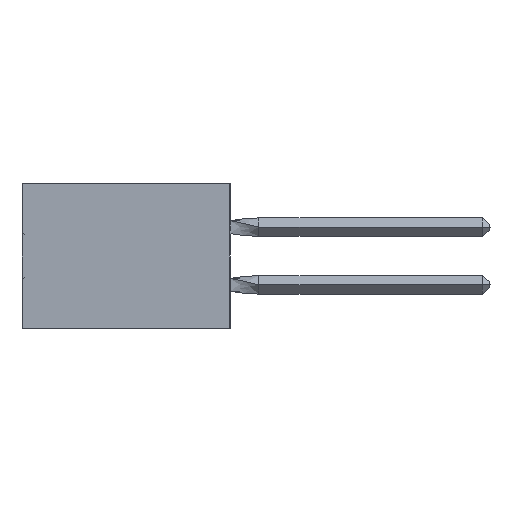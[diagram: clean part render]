
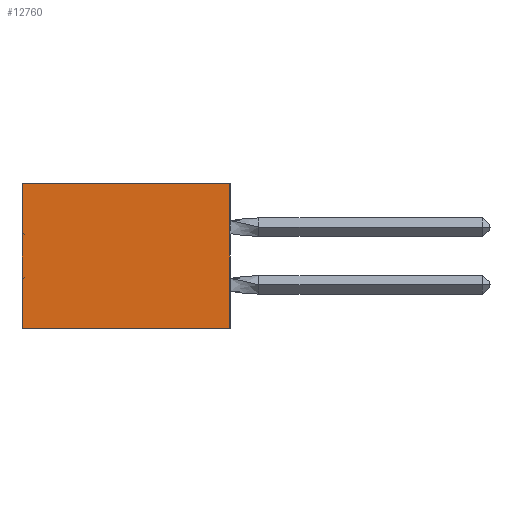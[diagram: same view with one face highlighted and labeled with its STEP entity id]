
A CAD part, left-side view. The second image highlights one B-rep face of the part: STEP entity #12760.
In plain terms, the highlighted planar face has unit normal (-1, 0, 0).
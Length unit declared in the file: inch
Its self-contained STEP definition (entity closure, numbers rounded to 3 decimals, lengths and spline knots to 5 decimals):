
#2190 = DIRECTION ( 'NONE',  ( 0., 0., -1. ) ) ;
#2735 = ORIENTED_EDGE ( 'NONE', *, *, #40915, .T. ) ;
#3404 = CARTESIAN_POINT ( 'NONE',  ( 0.305, 0., -0.5 ) ) ;
#7098 = DIRECTION ( 'NONE',  ( 0., 1., 0. ) ) ;
#8967 = AXIS2_PLACEMENT_3D ( 'NONE', #16172, #21092, #47996 ) ;
#10071 = FACE_OUTER_BOUND ( 'NONE', #18537, .T. ) ;
#10903 = VECTOR ( 'NONE', #37536, 39.37008 ) ;
#11004 = ORIENTED_EDGE ( 'NONE', *, *, #40364, .T. ) ;
#11494 = LINE ( 'NONE', #42683, #10903 ) ;
#12760 = ADVANCED_FACE ( 'NONE', ( #10071 ), #43999, .F. ) ;
#14700 = EDGE_CURVE ( 'NONE', #43816, #18410, #11494, .T. ) ;
#16172 = CARTESIAN_POINT ( 'NONE',  ( 0.305, 0., -0.5 ) ) ;
#18410 = VERTEX_POINT ( 'NONE', #3404 ) ;
#18537 = EDGE_LOOP ( 'NONE', ( #2735, #52264, #54970, #11004 ) ) ;
#19481 = VERTEX_POINT ( 'NONE', #58832 ) ;
#21092 = DIRECTION ( 'NONE',  ( 1., 0., 0. ) ) ;
#22545 = CARTESIAN_POINT ( 'NONE',  ( 0.305, 0., -0.5 ) ) ;
#24602 = VECTOR ( 'NONE', #2190, 39.37008 ) ;
#26042 = LINE ( 'NONE', #52566, #24602 ) ;
#26860 = LINE ( 'NONE', #57378, #36064 ) ;
#28786 = VERTEX_POINT ( 'NONE', #59001 ) ;
#36064 = VECTOR ( 'NONE', #7098, 39.37008 ) ;
#37536 = DIRECTION ( 'NONE',  ( 0., 0., -1. ) ) ;
#40364 = EDGE_CURVE ( 'NONE', #43816, #19481, #26860, .T. ) ;
#40915 = EDGE_CURVE ( 'NONE', #19481, #28786, #26042, .T. ) ;
#41258 = DIRECTION ( 'NONE',  ( 0., 1., 0. ) ) ;
#42683 = CARTESIAN_POINT ( 'NONE',  ( 0.305, 0., -0.5 ) ) ;
#43816 = VERTEX_POINT ( 'NONE', #46363 ) ;
#43999 = PLANE ( 'NONE',  #8967 ) ;
#45974 = EDGE_CURVE ( 'NONE', #18410, #28786, #54587, .T. ) ;
#46363 = CARTESIAN_POINT ( 'NONE',  ( 0.305, 0., 0. ) ) ;
#47996 = DIRECTION ( 'NONE',  ( 0., 0., -1. ) ) ;
#52264 = ORIENTED_EDGE ( 'NONE', *, *, #45974, .F. ) ;
#52566 = CARTESIAN_POINT ( 'NONE',  ( 0.305, 0.72, -0.5 ) ) ;
#54587 = LINE ( 'NONE', #22545, #58055 ) ;
#54970 = ORIENTED_EDGE ( 'NONE', *, *, #14700, .F. ) ;
#57378 = CARTESIAN_POINT ( 'NONE',  ( 0.305, 0., 0. ) ) ;
#58055 = VECTOR ( 'NONE', #41258, 39.37008 ) ;
#58832 = CARTESIAN_POINT ( 'NONE',  ( 0.305, 0.72, 0. ) ) ;
#59001 = CARTESIAN_POINT ( 'NONE',  ( 0.305, 0.72, -0.5 ) ) ;
